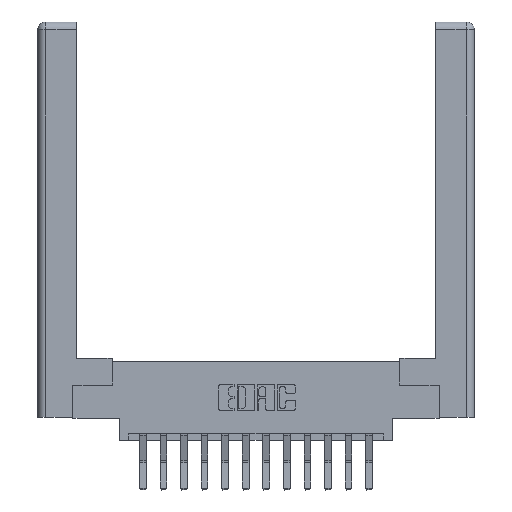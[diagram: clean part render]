
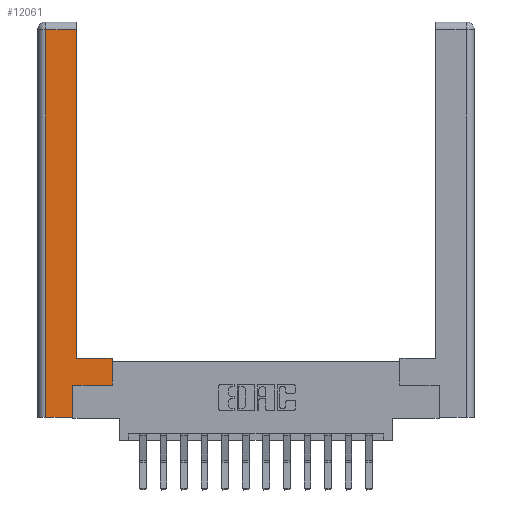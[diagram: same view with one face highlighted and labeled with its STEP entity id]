
A CAD part, top view. The second image highlights one B-rep face of the part: STEP entity #12061.
In plain terms, the highlighted planar face has unit normal (0, 0, 1).
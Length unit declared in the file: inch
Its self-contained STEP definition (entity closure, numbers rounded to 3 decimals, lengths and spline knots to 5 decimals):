
#127 = VECTOR ( 'NONE', #6515, 39.37008 ) ;
#303 = ORIENTED_EDGE ( 'NONE', *, *, #6152, .T. ) ;
#763 = CARTESIAN_POINT ( 'NONE',  ( 0.0615, 2.94, 0. ) ) ;
#1480 = EDGE_CURVE ( 'NONE', #10156, #2918, #14776, .T. ) ;
#2498 = VERTEX_POINT ( 'NONE', #5346 ) ;
#2855 = ORIENTED_EDGE ( 'NONE', *, *, #16025, .T. ) ;
#2876 = PLANE ( 'NONE',  #5730 ) ;
#2918 = VERTEX_POINT ( 'NONE', #3299 ) ;
#3150 = CARTESIAN_POINT ( 'NONE',  ( 0.265, 0.245, 0. ) ) ;
#3236 = EDGE_CURVE ( 'NONE', #2918, #4747, #10813, .T. ) ;
#3299 = CARTESIAN_POINT ( 'NONE',  ( 0.295, 2.94, 0. ) ) ;
#3831 = CARTESIAN_POINT ( 'NONE',  ( 0.265, 0., 0. ) ) ;
#3866 = CARTESIAN_POINT ( 'NONE',  ( 0.295, 0.45, 0. ) ) ;
#3900 = LINE ( 'NONE', #3150, #11229 ) ;
#4690 = VECTOR ( 'NONE', #13202, 39.37008 ) ;
#4705 = VECTOR ( 'NONE', #14005, 39.37008 ) ;
#4747 = VERTEX_POINT ( 'NONE', #16001 ) ;
#5100 = DIRECTION ( 'NONE',  ( -1., 0., 0. ) ) ;
#5148 = VECTOR ( 'NONE', #12009, 39.37008 ) ;
#5278 = CARTESIAN_POINT ( 'NONE',  ( 0.565, 0.45, 0. ) ) ;
#5346 = CARTESIAN_POINT ( 'NONE',  ( 0.0615, 0., 0. ) ) ;
#5404 = DIRECTION ( 'NONE',  ( 0., 0., -1. ) ) ;
#5502 = CARTESIAN_POINT ( 'NONE',  ( 0., 0., 0. ) ) ;
#5616 = EDGE_LOOP ( 'NONE', ( #10788, #14212, #303, #6406, #13303, #2855, #10227, #7109 ) ) ;
#5730 = AXIS2_PLACEMENT_3D ( 'NONE', #5502, #5404, #7813 ) ;
#5991 = VECTOR ( 'NONE', #15491, 39.37008 ) ;
#6057 = FACE_OUTER_BOUND ( 'NONE', #5616, .T. ) ;
#6152 = EDGE_CURVE ( 'NONE', #4747, #2498, #14657, .T. ) ;
#6406 = ORIENTED_EDGE ( 'NONE', *, *, #13028, .T. ) ;
#6515 = DIRECTION ( 'NONE',  ( 0., 1., 0. ) ) ;
#6658 = CARTESIAN_POINT ( 'NONE',  ( 0.295, 3., 0. ) ) ;
#7109 = ORIENTED_EDGE ( 'NONE', *, *, #14617, .T. ) ;
#7813 = DIRECTION ( 'NONE',  ( -1., 0., 0. ) ) ;
#8287 = LINE ( 'NONE', #3866, #10789 ) ;
#9012 = CARTESIAN_POINT ( 'NONE',  ( 0.565, 0.245, 0. ) ) ;
#9109 = CARTESIAN_POINT ( 'NONE',  ( 0.295, 0.45, 0. ) ) ;
#10156 = VERTEX_POINT ( 'NONE', #9109 ) ;
#10227 = ORIENTED_EDGE ( 'NONE', *, *, #11247, .T. ) ;
#10333 = VERTEX_POINT ( 'NONE', #9012 ) ;
#10482 = VERTEX_POINT ( 'NONE', #12576 ) ;
#10541 = DIRECTION ( 'NONE',  ( 0., 1., 0. ) ) ;
#10629 = VERTEX_POINT ( 'NONE', #3831 ) ;
#10788 = ORIENTED_EDGE ( 'NONE', *, *, #1480, .T. ) ;
#10789 = VECTOR ( 'NONE', #5100, 39.37008 ) ;
#10813 = LINE ( 'NONE', #763, #5991 ) ;
#10929 = LINE ( 'NONE', #13190, #5148 ) ;
#11229 = VECTOR ( 'NONE', #10541, 39.37008 ) ;
#11247 = EDGE_CURVE ( 'NONE', #10333, #14424, #12526, .T. ) ;
#11832 = CARTESIAN_POINT ( 'NONE',  ( 0.0615, 0., 0. ) ) ;
#12009 = DIRECTION ( 'NONE',  ( 1., 0., 0. ) ) ;
#12061 = ADVANCED_FACE ( 'NONE', ( #6057 ), #2876, .F. ) ;
#12526 = LINE ( 'NONE', #5278, #127 ) ;
#12576 = CARTESIAN_POINT ( 'NONE',  ( 0.265, 0.245, 0. ) ) ;
#13028 = EDGE_CURVE ( 'NONE', #2498, #10629, #15495, .T. ) ;
#13190 = CARTESIAN_POINT ( 'NONE',  ( 0.565, 0.245, 0. ) ) ;
#13202 = DIRECTION ( 'NONE',  ( 1., 0., 0. ) ) ;
#13205 = CARTESIAN_POINT ( 'NONE',  ( 0.565, 0.45, 0. ) ) ;
#13303 = ORIENTED_EDGE ( 'NONE', *, *, #13439, .T. ) ;
#13439 = EDGE_CURVE ( 'NONE', #10629, #10482, #3900, .T. ) ;
#13876 = VECTOR ( 'NONE', #14363, 39.37008 ) ;
#14005 = DIRECTION ( 'NONE',  ( 0., 1., 0. ) ) ;
#14212 = ORIENTED_EDGE ( 'NONE', *, *, #3236, .T. ) ;
#14273 = CARTESIAN_POINT ( 'NONE',  ( 0.265, 0., 0. ) ) ;
#14363 = DIRECTION ( 'NONE',  ( 0., -1., 0. ) ) ;
#14424 = VERTEX_POINT ( 'NONE', #13205 ) ;
#14617 = EDGE_CURVE ( 'NONE', #14424, #10156, #8287, .T. ) ;
#14657 = LINE ( 'NONE', #11832, #13876 ) ;
#14776 = LINE ( 'NONE', #6658, #4705 ) ;
#15491 = DIRECTION ( 'NONE',  ( -1., 0., 0. ) ) ;
#15495 = LINE ( 'NONE', #14273, #4690 ) ;
#16001 = CARTESIAN_POINT ( 'NONE',  ( 0.0615, 2.94, 0. ) ) ;
#16025 = EDGE_CURVE ( 'NONE', #10482, #10333, #10929, .T. ) ;
